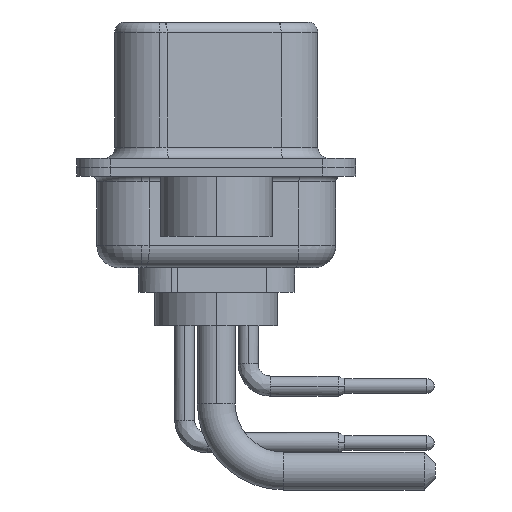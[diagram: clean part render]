
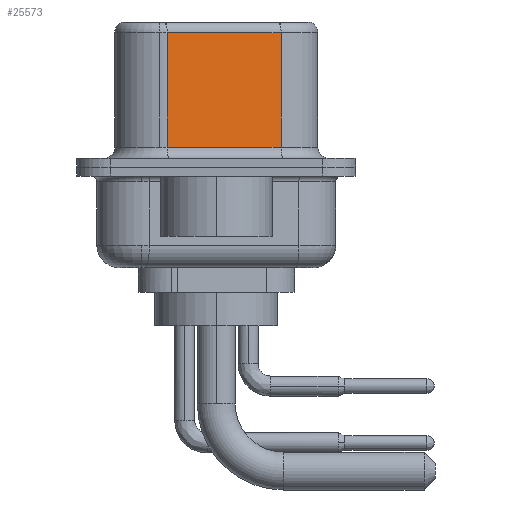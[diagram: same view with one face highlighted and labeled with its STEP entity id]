
A CAD part, left-side view. The second image highlights one B-rep face of the part: STEP entity #25573.
In plain terms, the highlighted planar face has unit normal (-0.985, -0.174, 0).
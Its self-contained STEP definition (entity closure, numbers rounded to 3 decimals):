
#710 = LINE ( 'NONE', #24724, #19288 ) ;
#843 = AXIS2_PLACEMENT_3D ( 'NONE', #20876, #16497, #6608 ) ;
#880 = LINE ( 'NONE', #7324, #4833 ) ;
#2904 = DIRECTION ( 'NONE',  ( 0., 0., -1. ) ) ;
#3045 = LINE ( 'NONE', #11473, #15893 ) ;
#4188 = VERTEX_POINT ( 'NONE', #5941 ) ;
#4587 = VERTEX_POINT ( 'NONE', #10680 ) ;
#4833 = VECTOR ( 'NONE', #14771, 1000. ) ;
#5005 = DIRECTION ( 'NONE',  ( 0.174, -0.985, 0. ) ) ;
#5941 = CARTESIAN_POINT ( 'NONE',  ( 3.68, 2.203, 0.9 ) ) ;
#6608 = DIRECTION ( 'NONE',  ( -0.174, 0.985, 0. ) ) ;
#6872 = FACE_OUTER_BOUND ( 'NONE', #21014, .T. ) ;
#7247 = VERTEX_POINT ( 'NONE', #16738 ) ;
#7324 = CARTESIAN_POINT ( 'NONE',  ( 4.58, -2.897, 6.02 ) ) ;
#8014 = CARTESIAN_POINT ( 'NONE',  ( 4.58, -2.897, 0.9 ) ) ;
#9009 = EDGE_CURVE ( 'NONE', #4587, #4188, #710, .T. ) ;
#9131 = EDGE_CURVE ( 'NONE', #7247, #15810, #20939, .T. ) ;
#10337 = EDGE_CURVE ( 'NONE', #7247, #4587, #880, .T. ) ;
#10429 = ORIENTED_EDGE ( 'NONE', *, *, #18825, .T. ) ;
#10680 = CARTESIAN_POINT ( 'NONE',  ( 3.68, 2.203, 6.02 ) ) ;
#11473 = CARTESIAN_POINT ( 'NONE',  ( 4.58, -2.897, 0.9 ) ) ;
#11747 = ORIENTED_EDGE ( 'NONE', *, *, #10337, .T. ) ;
#12580 = PLANE ( 'NONE',  #843 ) ;
#14354 = DIRECTION ( 'NONE',  ( 0., 0., -1. ) ) ;
#14771 = DIRECTION ( 'NONE',  ( -0.174, 0.985, 0. ) ) ;
#15153 = ORIENTED_EDGE ( 'NONE', *, *, #9009, .T. ) ;
#15810 = VERTEX_POINT ( 'NONE', #8014 ) ;
#15893 = VECTOR ( 'NONE', #5005, 1000. ) ;
#16497 = DIRECTION ( 'NONE',  ( 0.985, 0.174, 0. ) ) ;
#16599 = ORIENTED_EDGE ( 'NONE', *, *, #9131, .F. ) ;
#16738 = CARTESIAN_POINT ( 'NONE',  ( 4.58, -2.897, 6.02 ) ) ;
#17332 = VECTOR ( 'NONE', #2904, 1000. ) ;
#18825 = EDGE_CURVE ( 'NONE', #4188, #15810, #3045, .T. ) ;
#19288 = VECTOR ( 'NONE', #14354, 1000. ) ;
#20876 = CARTESIAN_POINT ( 'NONE',  ( 4.58, -2.897, 6.52 ) ) ;
#20939 = LINE ( 'NONE', #25216, #17332 ) ;
#21014 = EDGE_LOOP ( 'NONE', ( #16599, #11747, #15153, #10429 ) ) ;
#24724 = CARTESIAN_POINT ( 'NONE',  ( 3.68, 2.203, 6.52 ) ) ;
#25216 = CARTESIAN_POINT ( 'NONE',  ( 4.58, -2.897, 6.52 ) ) ;
#25573 = ADVANCED_FACE ( 'NONE', ( #6872 ), #12580, .F. ) ;
